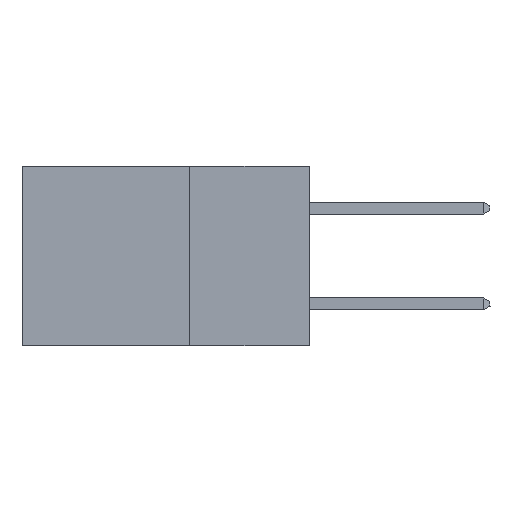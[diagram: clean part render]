
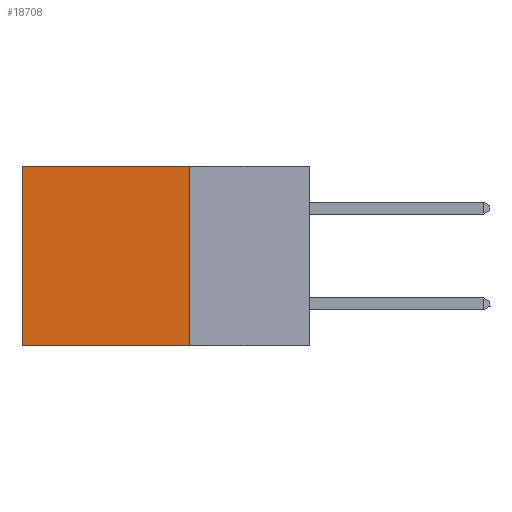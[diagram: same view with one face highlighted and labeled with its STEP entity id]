
A CAD part, left-side view. The second image highlights one B-rep face of the part: STEP entity #18708.
In plain terms, the highlighted planar face has unit normal (-1, 0, 0).
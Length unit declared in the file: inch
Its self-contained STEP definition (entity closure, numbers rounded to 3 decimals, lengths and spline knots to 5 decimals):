
#273 = CARTESIAN_POINT ( 'NONE',  ( 0.2875, 0.6, -0.375 ) ) ;
#818 = FACE_OUTER_BOUND ( 'NONE', #4035, .T. ) ;
#942 = DIRECTION ( 'NONE',  ( 1., 0., 0. ) ) ;
#1244 = DIRECTION ( 'NONE',  ( 0., 1., 0. ) ) ;
#1591 = DIRECTION ( 'NONE',  ( 0., 0., -1. ) ) ;
#1974 = CARTESIAN_POINT ( 'NONE',  ( 0.2875, 0.25, -0.375 ) ) ;
#2321 = LINE ( 'NONE', #2878, #15048 ) ;
#2878 = CARTESIAN_POINT ( 'NONE',  ( 0.2875, 0.25, -0.375 ) ) ;
#3181 = DIRECTION ( 'NONE',  ( 0., 0., -1. ) ) ;
#3599 = CARTESIAN_POINT ( 'NONE',  ( 0.2875, 0.6, 0. ) ) ;
#3735 = DIRECTION ( 'NONE',  ( 0., 0., -1. ) ) ;
#4035 = EDGE_LOOP ( 'NONE', ( #10160, #9668, #13575, #13380 ) ) ;
#4844 = PLANE ( 'NONE',  #16693 ) ;
#7534 = CARTESIAN_POINT ( 'NONE',  ( 0.2875, 0.25, 0. ) ) ;
#7773 = EDGE_CURVE ( 'NONE', #16272, #11709, #17127, .T. ) ;
#7828 = DIRECTION ( 'NONE',  ( 0., 1., 0. ) ) ;
#8857 = CARTESIAN_POINT ( 'NONE',  ( 0.2875, 0.6, -0.375 ) ) ;
#9074 = LINE ( 'NONE', #273, #9978 ) ;
#9229 = VECTOR ( 'NONE', #1591, 39.37008 ) ;
#9549 = EDGE_CURVE ( 'NONE', #11709, #18045, #2321, .T. ) ;
#9668 = ORIENTED_EDGE ( 'NONE', *, *, #9549, .F. ) ;
#9978 = VECTOR ( 'NONE', #3181, 39.37008 ) ;
#10160 = ORIENTED_EDGE ( 'NONE', *, *, #14289, .T. ) ;
#11709 = VERTEX_POINT ( 'NONE', #15145 ) ;
#13380 = ORIENTED_EDGE ( 'NONE', *, *, #15143, .T. ) ;
#13422 = CARTESIAN_POINT ( 'NONE',  ( 0.2875, 0.25, -0.375 ) ) ;
#13575 = ORIENTED_EDGE ( 'NONE', *, *, #7773, .F. ) ;
#13799 = VECTOR ( 'NONE', #7828, 39.37008 ) ;
#14251 = LINE ( 'NONE', #18020, #13799 ) ;
#14289 = EDGE_CURVE ( 'NONE', #14873, #18045, #9074, .T. ) ;
#14873 = VERTEX_POINT ( 'NONE', #3599 ) ;
#15048 = VECTOR ( 'NONE', #1244, 39.37008 ) ;
#15143 = EDGE_CURVE ( 'NONE', #16272, #14873, #14251, .T. ) ;
#15145 = CARTESIAN_POINT ( 'NONE',  ( 0.2875, 0.25, -0.375 ) ) ;
#16272 = VERTEX_POINT ( 'NONE', #7534 ) ;
#16693 = AXIS2_PLACEMENT_3D ( 'NONE', #1974, #942, #3735 ) ;
#17127 = LINE ( 'NONE', #13422, #9229 ) ;
#18020 = CARTESIAN_POINT ( 'NONE',  ( 0.2875, 0.25, 0. ) ) ;
#18045 = VERTEX_POINT ( 'NONE', #8857 ) ;
#18708 = ADVANCED_FACE ( 'NONE', ( #818 ), #4844, .F. ) ;
